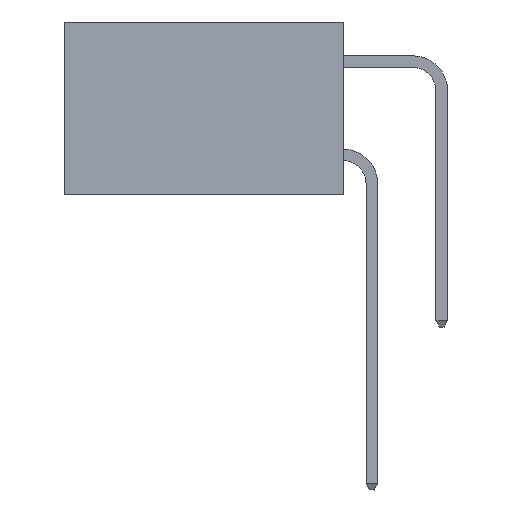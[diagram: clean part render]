
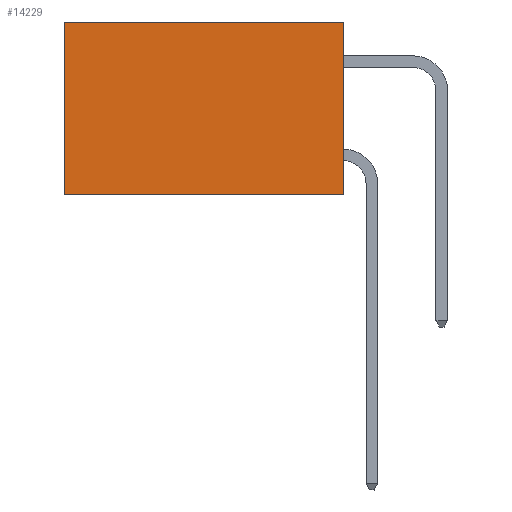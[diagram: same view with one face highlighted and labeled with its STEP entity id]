
A CAD part, left-side view. The second image highlights one B-rep face of the part: STEP entity #14229.
In plain terms, the highlighted planar face has unit normal (-1, 0, 0).
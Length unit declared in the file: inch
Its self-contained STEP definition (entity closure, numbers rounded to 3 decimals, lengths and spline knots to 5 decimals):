
#1142 = CARTESIAN_POINT ( 'NONE',  ( 0.298, 0.6, 0. ) ) ;
#1289 = DIRECTION ( 'NONE',  ( 0., 0., -1. ) ) ;
#1541 = CARTESIAN_POINT ( 'NONE',  ( 0.298, 0.6, 0. ) ) ;
#2088 = DIRECTION ( 'NONE',  ( 0., 1., 0. ) ) ;
#2139 = LINE ( 'NONE', #4970, #14111 ) ;
#2443 = EDGE_LOOP ( 'NONE', ( #15063, #11262, #17896, #18339 ) ) ;
#2818 = CARTESIAN_POINT ( 'NONE',  ( 0.298, 0., -0.37 ) ) ;
#2991 = CARTESIAN_POINT ( 'NONE',  ( 0.298, 0.6, -0.37 ) ) ;
#3303 = DIRECTION ( 'NONE',  ( 0., 1., 0. ) ) ;
#3931 = CARTESIAN_POINT ( 'NONE',  ( 0.298, 0., 0. ) ) ;
#4165 = CARTESIAN_POINT ( 'NONE',  ( 0.298, 0., 0. ) ) ;
#4581 = VECTOR ( 'NONE', #8782, 39.37008 ) ;
#4766 = EDGE_CURVE ( 'NONE', #19202, #9715, #14932, .T. ) ;
#4970 = CARTESIAN_POINT ( 'NONE',  ( 0.298, 0., 0. ) ) ;
#8782 = DIRECTION ( 'NONE',  ( 0., 0., -1. ) ) ;
#9715 = VERTEX_POINT ( 'NONE', #2991 ) ;
#9784 = CARTESIAN_POINT ( 'NONE',  ( 0.298, 0., 0. ) ) ;
#11133 = LINE ( 'NONE', #16266, #17624 ) ;
#11153 = EDGE_CURVE ( 'NONE', #11328, #9715, #11133, .T. ) ;
#11262 = ORIENTED_EDGE ( 'NONE', *, *, #11153, .F. ) ;
#11328 = VERTEX_POINT ( 'NONE', #2818 ) ;
#11549 = DIRECTION ( 'NONE',  ( 0., 0., -1. ) ) ;
#11835 = AXIS2_PLACEMENT_3D ( 'NONE', #9784, #16905, #11549 ) ;
#13450 = VECTOR ( 'NONE', #1289, 39.37008 ) ;
#13554 = LINE ( 'NONE', #3931, #4581 ) ;
#14111 = VECTOR ( 'NONE', #3303, 39.37008 ) ;
#14229 = ADVANCED_FACE ( 'NONE', ( #21000 ), #20147, .F. ) ;
#14932 = LINE ( 'NONE', #1142, #13450 ) ;
#15063 = ORIENTED_EDGE ( 'NONE', *, *, #4766, .T. ) ;
#16157 = VERTEX_POINT ( 'NONE', #4165 ) ;
#16266 = CARTESIAN_POINT ( 'NONE',  ( 0.298, 0., -0.37 ) ) ;
#16905 = DIRECTION ( 'NONE',  ( 1., 0., 0. ) ) ;
#17624 = VECTOR ( 'NONE', #2088, 39.37008 ) ;
#17896 = ORIENTED_EDGE ( 'NONE', *, *, #18095, .F. ) ;
#18095 = EDGE_CURVE ( 'NONE', #16157, #11328, #13554, .T. ) ;
#18339 = ORIENTED_EDGE ( 'NONE', *, *, #18452, .T. ) ;
#18452 = EDGE_CURVE ( 'NONE', #16157, #19202, #2139, .T. ) ;
#19202 = VERTEX_POINT ( 'NONE', #1541 ) ;
#20147 = PLANE ( 'NONE',  #11835 ) ;
#21000 = FACE_OUTER_BOUND ( 'NONE', #2443, .T. ) ;
